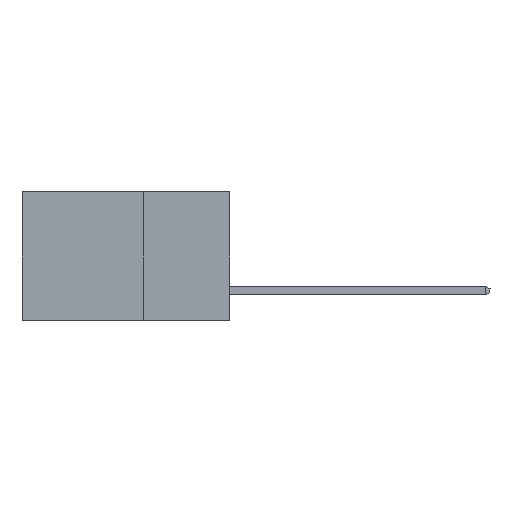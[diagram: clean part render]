
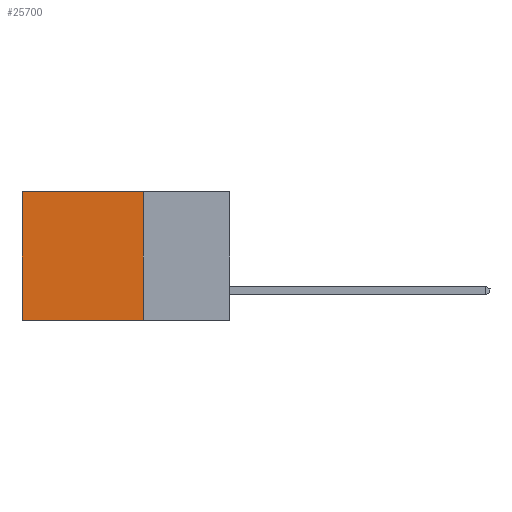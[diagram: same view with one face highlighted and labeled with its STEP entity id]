
A CAD part, left-side view. The second image highlights one B-rep face of the part: STEP entity #25700.
In plain terms, the highlighted planar face has unit normal (-1, 0, 0).
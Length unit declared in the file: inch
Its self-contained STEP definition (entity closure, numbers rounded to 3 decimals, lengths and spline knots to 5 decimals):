
#80 = VERTEX_POINT ( 'NONE', #6297 ) ;
#1078 = VECTOR ( 'NONE', #13751, 39.37008 ) ;
#1302 = LINE ( 'NONE', #23183, #10590 ) ;
#2080 = CARTESIAN_POINT ( 'NONE',  ( 0.2615, 0.25, -0.37 ) ) ;
#2952 = CARTESIAN_POINT ( 'NONE',  ( 0.2615, 0.25, -0.37 ) ) ;
#3124 = DIRECTION ( 'NONE',  ( 1., 0., 0. ) ) ;
#3896 = EDGE_CURVE ( 'NONE', #8806, #12155, #12134, .T. ) ;
#5380 = AXIS2_PLACEMENT_3D ( 'NONE', #22930, #3124, #11061 ) ;
#5757 = CARTESIAN_POINT ( 'NONE',  ( 0.2615, 0.6, 0. ) ) ;
#6297 = CARTESIAN_POINT ( 'NONE',  ( 0.2615, 0.25, 0. ) ) ;
#7972 = DIRECTION ( 'NONE',  ( 0., 0., -1. ) ) ;
#8100 = CARTESIAN_POINT ( 'NONE',  ( 0.2615, 0.6, -0.37 ) ) ;
#8156 = VECTOR ( 'NONE', #16382, 39.37008 ) ;
#8211 = ORIENTED_EDGE ( 'NONE', *, *, #3896, .T. ) ;
#8806 = VERTEX_POINT ( 'NONE', #5757 ) ;
#10590 = VECTOR ( 'NONE', #23561, 39.37008 ) ;
#11061 = DIRECTION ( 'NONE',  ( 0., 0., -1. ) ) ;
#12042 = CARTESIAN_POINT ( 'NONE',  ( 0.2615, 0.25, 0. ) ) ;
#12134 = LINE ( 'NONE', #8100, #12451 ) ;
#12155 = VERTEX_POINT ( 'NONE', #16669 ) ;
#12310 = EDGE_CURVE ( 'NONE', #80, #22969, #1302, .T. ) ;
#12451 = VECTOR ( 'NONE', #7972, 39.37008 ) ;
#13751 = DIRECTION ( 'NONE',  ( 0., 1., 0. ) ) ;
#14889 = ORIENTED_EDGE ( 'NONE', *, *, #18570, .T. ) ;
#16382 = DIRECTION ( 'NONE',  ( 0., 1., 0. ) ) ;
#16555 = ORIENTED_EDGE ( 'NONE', *, *, #21343, .F. ) ;
#16669 = CARTESIAN_POINT ( 'NONE',  ( 0.2615, 0.6, -0.37 ) ) ;
#17545 = ORIENTED_EDGE ( 'NONE', *, *, #12310, .F. ) ;
#18570 = EDGE_CURVE ( 'NONE', #80, #8806, #25597, .T. ) ;
#21105 = PLANE ( 'NONE',  #5380 ) ;
#21343 = EDGE_CURVE ( 'NONE', #22969, #12155, #22134, .T. ) ;
#22134 = LINE ( 'NONE', #2080, #8156 ) ;
#22930 = CARTESIAN_POINT ( 'NONE',  ( 0.2615, 0.25, -0.37 ) ) ;
#22969 = VERTEX_POINT ( 'NONE', #2952 ) ;
#23168 = EDGE_LOOP ( 'NONE', ( #8211, #16555, #17545, #14889 ) ) ;
#23183 = CARTESIAN_POINT ( 'NONE',  ( 0.2615, 0.25, -0.37 ) ) ;
#23561 = DIRECTION ( 'NONE',  ( 0., 0., -1. ) ) ;
#25127 = FACE_OUTER_BOUND ( 'NONE', #23168, .T. ) ;
#25597 = LINE ( 'NONE', #12042, #1078 ) ;
#25700 = ADVANCED_FACE ( 'NONE', ( #25127 ), #21105, .F. ) ;
